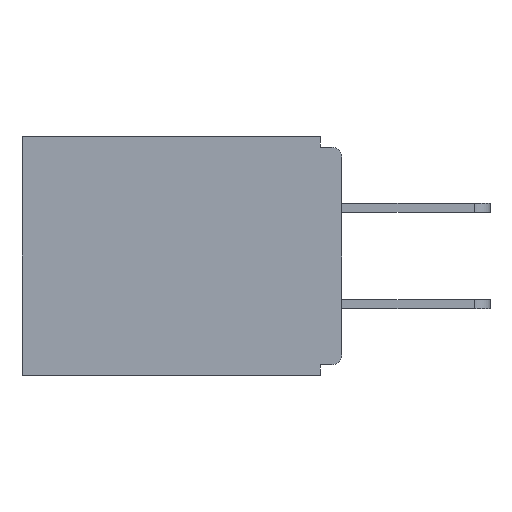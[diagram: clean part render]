
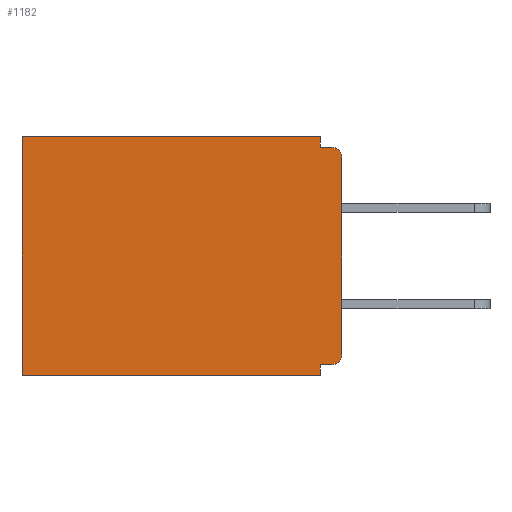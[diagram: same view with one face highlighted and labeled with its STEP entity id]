
A CAD part, left-side view. The second image highlights one B-rep face of the part: STEP entity #1182.
In plain terms, the highlighted planar face has unit normal (-1, 0, 0).
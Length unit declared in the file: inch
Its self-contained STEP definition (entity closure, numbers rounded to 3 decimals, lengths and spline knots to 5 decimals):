
#7 = ORIENTED_EDGE ( 'NONE', *, *, #9704, .F. ) ;
#184 = LINE ( 'NONE', #3322, #1951 ) ;
#366 = LINE ( 'NONE', #7158, #974 ) ;
#603 = LINE ( 'NONE', #5591, #1097 ) ;
#624 = LINE ( 'NONE', #642, #1483 ) ;
#642 = CARTESIAN_POINT ( 'NONE',  ( 0.298, 0., -0.343 ) ) ;
#884 = ORIENTED_EDGE ( 'NONE', *, *, #1670, .T. ) ;
#974 = VECTOR ( 'NONE', #3987, 39.37008 ) ;
#1097 = VECTOR ( 'NONE', #2223, 39.37008 ) ;
#1111 = CARTESIAN_POINT ( 'NONE',  ( 0.298, 0., 0. ) ) ;
#1182 = ADVANCED_FACE ( 'NONE', ( #10128 ), #9941, .F. ) ;
#1418 = AXIS2_PLACEMENT_3D ( 'NONE', #7271, #2417, #9604 ) ;
#1483 = VECTOR ( 'NONE', #2297, 39.37008 ) ;
#1670 = EDGE_CURVE ( 'NONE', #2501, #9193, #7593, .T. ) ;
#1951 = VECTOR ( 'NONE', #5759, 39.37008 ) ;
#2034 = CARTESIAN_POINT ( 'NONE',  ( 0.298, 0., -0.03 ) ) ;
#2046 = LINE ( 'NONE', #8414, #5359 ) ;
#2223 = DIRECTION ( 'NONE',  ( 0., 0., -1. ) ) ;
#2276 = VERTEX_POINT ( 'NONE', #2295 ) ;
#2289 = EDGE_CURVE ( 'NONE', #8107, #10325, #366, .T. ) ;
#2295 = CARTESIAN_POINT ( 'NONE',  ( 0.298, 0.031, -0.015 ) ) ;
#2297 = DIRECTION ( 'NONE',  ( 0., 1., 0. ) ) ;
#2361 = DIRECTION ( 'NONE',  ( 0., -1., 0. ) ) ;
#2417 = DIRECTION ( 'NONE',  ( -1., 0., 0. ) ) ;
#2497 = CARTESIAN_POINT ( 'NONE',  ( 0.298, 0.031, 0. ) ) ;
#2501 = VERTEX_POINT ( 'NONE', #2497 ) ;
#2694 = VERTEX_POINT ( 'NONE', #3651 ) ;
#2931 = CARTESIAN_POINT ( 'NONE',  ( 0.298, 0.46, 0. ) ) ;
#3215 = EDGE_CURVE ( 'NONE', #5900, #9876, #3780, .T. ) ;
#3276 = ORIENTED_EDGE ( 'NONE', *, *, #3215, .T. ) ;
#3322 = CARTESIAN_POINT ( 'NONE',  ( 0.298, 0., 0. ) ) ;
#3596 = VERTEX_POINT ( 'NONE', #9423 ) ;
#3651 = CARTESIAN_POINT ( 'NONE',  ( 0.298, 0.015, -0.015 ) ) ;
#3745 = VECTOR ( 'NONE', #2361, 39.37008 ) ;
#3780 = CIRCLE ( 'NONE', #1418, 0.015 ) ;
#3987 = DIRECTION ( 'NONE',  ( 0., 0., -1. ) ) ;
#4027 = ORIENTED_EDGE ( 'NONE', *, *, #4849, .T. ) ;
#4383 = DIRECTION ( 'NONE',  ( 0., 1., 0. ) ) ;
#4431 = CARTESIAN_POINT ( 'NONE',  ( 0.298, 0.031, -0.328 ) ) ;
#4565 = CARTESIAN_POINT ( 'NONE',  ( 0.298, 0.031, -0.343 ) ) ;
#4776 = DIRECTION ( 'NONE',  ( -1., 0., 0. ) ) ;
#4816 = AXIS2_PLACEMENT_3D ( 'NONE', #1111, #6836, #5175 ) ;
#4849 = EDGE_CURVE ( 'NONE', #9193, #3596, #603, .T. ) ;
#5119 = AXIS2_PLACEMENT_3D ( 'NONE', #10442, #4776, #5643 ) ;
#5169 = DIRECTION ( 'NONE',  ( 0., 1., 0. ) ) ;
#5175 = DIRECTION ( 'NONE',  ( 0., 0., -1. ) ) ;
#5216 = VERTEX_POINT ( 'NONE', #2034 ) ;
#5297 = CARTESIAN_POINT ( 'NONE',  ( 0.298, 0., 0. ) ) ;
#5337 = EDGE_CURVE ( 'NONE', #2501, #2276, #8183, .T. ) ;
#5359 = VECTOR ( 'NONE', #5169, 39.37008 ) ;
#5577 = ORIENTED_EDGE ( 'NONE', *, *, #8113, .F. ) ;
#5591 = CARTESIAN_POINT ( 'NONE',  ( 0.298, 0.46, 0. ) ) ;
#5643 = DIRECTION ( 'NONE',  ( 0., 0., -1. ) ) ;
#5759 = DIRECTION ( 'NONE',  ( 0., 0., -1. ) ) ;
#5900 = VERTEX_POINT ( 'NONE', #7203 ) ;
#6198 = DIRECTION ( 'NONE',  ( 0., 0., -1. ) ) ;
#6552 = ORIENTED_EDGE ( 'NONE', *, *, #9260, .T. ) ;
#6557 = EDGE_CURVE ( 'NONE', #2276, #2694, #9675, .T. ) ;
#6679 = EDGE_CURVE ( 'NONE', #5216, #9876, #184, .T. ) ;
#6836 = DIRECTION ( 'NONE',  ( 1., 0., 0. ) ) ;
#7124 = ORIENTED_EDGE ( 'NONE', *, *, #5337, .F. ) ;
#7158 = CARTESIAN_POINT ( 'NONE',  ( 0.298, 0.031, -0.343 ) ) ;
#7203 = CARTESIAN_POINT ( 'NONE',  ( 0.298, 0.015, -0.328 ) ) ;
#7212 = CARTESIAN_POINT ( 'NONE',  ( 0.298, 0., -0.015 ) ) ;
#7271 = CARTESIAN_POINT ( 'NONE',  ( 0.298, 0.015, -0.313 ) ) ;
#7344 = CIRCLE ( 'NONE', #5119, 0.015 ) ;
#7593 = LINE ( 'NONE', #5297, #9492 ) ;
#8107 = VERTEX_POINT ( 'NONE', #4431 ) ;
#8113 = EDGE_CURVE ( 'NONE', #5900, #8107, #2046, .T. ) ;
#8183 = LINE ( 'NONE', #4565, #8576 ) ;
#8414 = CARTESIAN_POINT ( 'NONE',  ( 0.298, 0., -0.328 ) ) ;
#8465 = EDGE_LOOP ( 'NONE', ( #6552, #8606, #7124, #884, #4027, #7, #8584, #5577, #3276, #10418 ) ) ;
#8576 = VECTOR ( 'NONE', #6198, 39.37008 ) ;
#8584 = ORIENTED_EDGE ( 'NONE', *, *, #2289, .F. ) ;
#8606 = ORIENTED_EDGE ( 'NONE', *, *, #6557, .F. ) ;
#8837 = CARTESIAN_POINT ( 'NONE',  ( 0.298, 0., -0.313 ) ) ;
#9193 = VERTEX_POINT ( 'NONE', #2931 ) ;
#9260 = EDGE_CURVE ( 'NONE', #5216, #2694, #7344, .T. ) ;
#9329 = CARTESIAN_POINT ( 'NONE',  ( 0.298, 0.031, -0.343 ) ) ;
#9423 = CARTESIAN_POINT ( 'NONE',  ( 0.298, 0.46, -0.343 ) ) ;
#9492 = VECTOR ( 'NONE', #4383, 39.37008 ) ;
#9604 = DIRECTION ( 'NONE',  ( 0., 0., -1. ) ) ;
#9675 = LINE ( 'NONE', #7212, #3745 ) ;
#9704 = EDGE_CURVE ( 'NONE', #10325, #3596, #624, .T. ) ;
#9876 = VERTEX_POINT ( 'NONE', #8837 ) ;
#9941 = PLANE ( 'NONE',  #4816 ) ;
#10128 = FACE_OUTER_BOUND ( 'NONE', #8465, .T. ) ;
#10325 = VERTEX_POINT ( 'NONE', #9329 ) ;
#10418 = ORIENTED_EDGE ( 'NONE', *, *, #6679, .F. ) ;
#10442 = CARTESIAN_POINT ( 'NONE',  ( 0.298, 0.015, -0.03 ) ) ;
